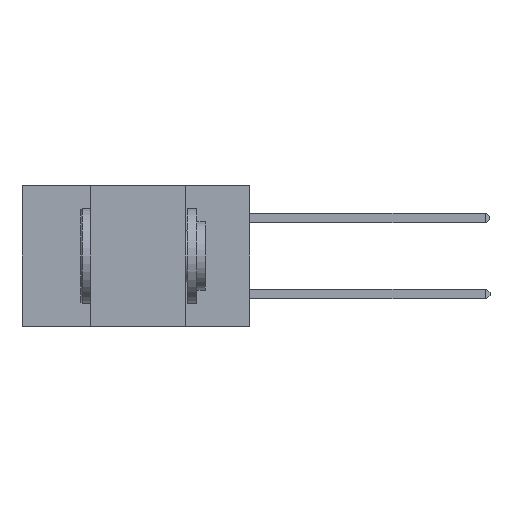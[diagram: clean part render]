
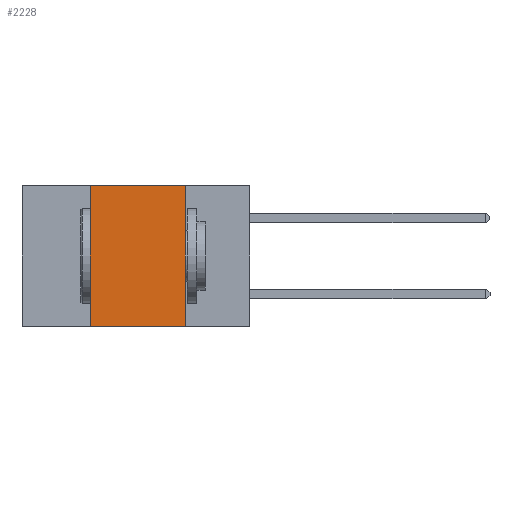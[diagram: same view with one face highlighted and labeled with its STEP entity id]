
A CAD part, left-side view. The second image highlights one B-rep face of the part: STEP entity #2228.
In plain terms, the highlighted planar face has unit normal (-1, 0, 0).
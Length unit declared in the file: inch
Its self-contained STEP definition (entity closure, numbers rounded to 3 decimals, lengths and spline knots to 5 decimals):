
#648 = DIRECTION ( 'NONE',  ( 0., 0., -1. ) ) ;
#1103 = LINE ( 'NONE', #7642, #19747 ) ;
#2033 = ORIENTED_EDGE ( 'NONE', *, *, #11459, .T. ) ;
#2228 = ADVANCED_FACE ( 'NONE', ( #16453 ), #20435, .F. ) ;
#2324 = EDGE_CURVE ( 'NONE', #18273, #17694, #22839, .T. ) ;
#2628 = CARTESIAN_POINT ( 'NONE',  ( 0., 0.42, 0. ) ) ;
#2828 = VERTEX_POINT ( 'NONE', #11180 ) ;
#3594 = EDGE_CURVE ( 'NONE', #13742, #2828, #4553, .T. ) ;
#4553 = LINE ( 'NONE', #17967, #13092 ) ;
#5546 = ORIENTED_EDGE ( 'NONE', *, *, #3594, .F. ) ;
#7342 = EDGE_LOOP ( 'NONE', ( #5546, #17599, #15660, #2033 ) ) ;
#7642 = CARTESIAN_POINT ( 'NONE',  ( 0., 0.6, -0.37 ) ) ;
#8516 = VECTOR ( 'NONE', #10923, 39.37008 ) ;
#10162 = CARTESIAN_POINT ( 'NONE',  ( 0., 0.17, 0. ) ) ;
#10923 = DIRECTION ( 'NONE',  ( 0., -1., 0. ) ) ;
#11180 = CARTESIAN_POINT ( 'NONE',  ( 0., 0.17, -0.37 ) ) ;
#11459 = EDGE_CURVE ( 'NONE', #18273, #2828, #1103, .T. ) ;
#12661 = CARTESIAN_POINT ( 'NONE',  ( 0., 0.6, 0. ) ) ;
#12688 = AXIS2_PLACEMENT_3D ( 'NONE', #20413, #20405, #20385 ) ;
#13092 = VECTOR ( 'NONE', #648, 39.37008 ) ;
#13299 = LINE ( 'NONE', #12661, #8516 ) ;
#13508 = CARTESIAN_POINT ( 'NONE',  ( 0., 0.42, -0.37 ) ) ;
#13742 = VERTEX_POINT ( 'NONE', #10162 ) ;
#14853 = DIRECTION ( 'NONE',  ( 0., -1., 0. ) ) ;
#15660 = ORIENTED_EDGE ( 'NONE', *, *, #2324, .F. ) ;
#16453 = FACE_OUTER_BOUND ( 'NONE', #7342, .T. ) ;
#17599 = ORIENTED_EDGE ( 'NONE', *, *, #21774, .F. ) ;
#17694 = VERTEX_POINT ( 'NONE', #2628 ) ;
#17967 = CARTESIAN_POINT ( 'NONE',  ( 0., 0.17, 0. ) ) ;
#18273 = VERTEX_POINT ( 'NONE', #13508 ) ;
#18324 = VECTOR ( 'NONE', #18911, 39.37008 ) ;
#18911 = DIRECTION ( 'NONE',  ( 0., 0., 1. ) ) ;
#19002 = CARTESIAN_POINT ( 'NONE',  ( 0., 0.42, 0. ) ) ;
#19747 = VECTOR ( 'NONE', #14853, 39.37008 ) ;
#20385 = DIRECTION ( 'NONE',  ( 0., 0., -1. ) ) ;
#20405 = DIRECTION ( 'NONE',  ( 1., 0., 0. ) ) ;
#20413 = CARTESIAN_POINT ( 'NONE',  ( 0., 0.6, 0. ) ) ;
#20435 = PLANE ( 'NONE',  #12688 ) ;
#21774 = EDGE_CURVE ( 'NONE', #17694, #13742, #13299, .T. ) ;
#22839 = LINE ( 'NONE', #19002, #18324 ) ;
